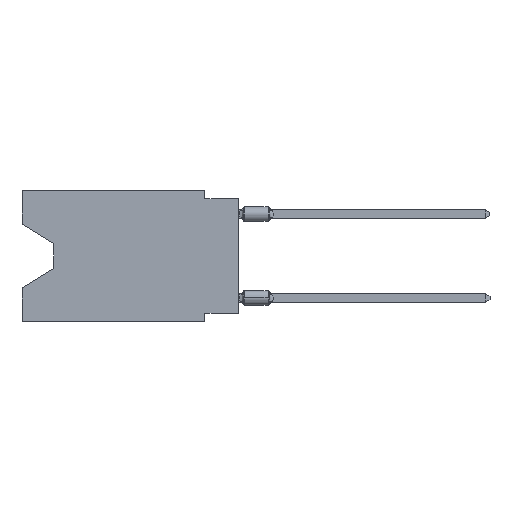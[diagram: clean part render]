
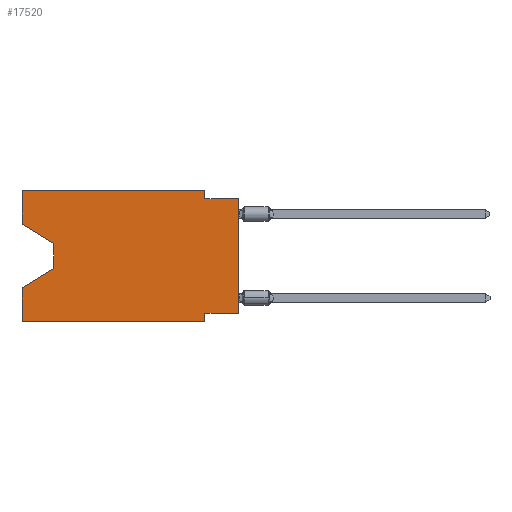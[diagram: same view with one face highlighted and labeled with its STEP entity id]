
A CAD part, left-side view. The second image highlights one B-rep face of the part: STEP entity #17520.
In plain terms, the highlighted planar face has unit normal (-1, 0, 0).
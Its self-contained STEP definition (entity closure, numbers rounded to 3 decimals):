
#635 = CARTESIAN_POINT ( 'NONE',  ( 0., 13.97, -5.893 ) ) ;
#1860 = CARTESIAN_POINT ( 'NONE',  ( 0., 0., 0. ) ) ;
#1913 = LINE ( 'NONE', #5358, #4241 ) ;
#2223 = CARTESIAN_POINT ( 'NONE',  ( 0., 16.383, -9.906 ) ) ;
#2336 = DIRECTION ( 'NONE',  ( 0., -1., 0. ) ) ;
#2505 = DIRECTION ( 'NONE',  ( 0., 0., 1. ) ) ;
#2798 = VECTOR ( 'NONE', #19032, 1000. ) ;
#3172 = ORIENTED_EDGE ( 'NONE', *, *, #19036, .T. ) ;
#3217 = EDGE_CURVE ( 'NONE', #8959, #5045, #1913, .T. ) ;
#3568 = DIRECTION ( 'NONE',  ( 0., -1., 0. ) ) ;
#4062 = DIRECTION ( 'NONE',  ( 1., 0., 0. ) ) ;
#4241 = VECTOR ( 'NONE', #5244, 1000. ) ;
#4574 = CARTESIAN_POINT ( 'NONE',  ( 0., 2.54, -9.906 ) ) ;
#4820 = CARTESIAN_POINT ( 'NONE',  ( 0., 13.97, -5.893 ) ) ;
#4947 = EDGE_CURVE ( 'NONE', #20258, #6249, #11176, .T. ) ;
#5045 = VERTEX_POINT ( 'NONE', #15097 ) ;
#5244 = DIRECTION ( 'NONE',  ( 0., 0., -1. ) ) ;
#5317 = VERTEX_POINT ( 'NONE', #7220 ) ;
#5358 = CARTESIAN_POINT ( 'NONE',  ( 0., 2.54, 0. ) ) ;
#5420 = LINE ( 'NONE', #1860, #16963 ) ;
#5758 = VECTOR ( 'NONE', #14984, 1000. ) ;
#5799 = PLANE ( 'NONE',  #7624 ) ;
#5903 = CARTESIAN_POINT ( 'NONE',  ( 0., 13.97, -4.013 ) ) ;
#6205 = VERTEX_POINT ( 'NONE', #11636 ) ;
#6249 = VERTEX_POINT ( 'NONE', #9445 ) ;
#6511 = CARTESIAN_POINT ( 'NONE',  ( 0., 16.383, -7.36 ) ) ;
#7022 = LINE ( 'NONE', #19379, #10149 ) ;
#7165 = CARTESIAN_POINT ( 'NONE',  ( 0., 0., -9.271 ) ) ;
#7220 = CARTESIAN_POINT ( 'NONE',  ( 0., 16.383, -2.546 ) ) ;
#7221 = VECTOR ( 'NONE', #15803, 1000. ) ;
#7257 = CARTESIAN_POINT ( 'NONE',  ( 0., 0., -0.635 ) ) ;
#7326 = VECTOR ( 'NONE', #2336, 1000. ) ;
#7369 = EDGE_CURVE ( 'NONE', #6205, #18120, #13183, .T. ) ;
#7464 = EDGE_CURVE ( 'NONE', #16154, #20258, #20544, .T. ) ;
#7595 = ORIENTED_EDGE ( 'NONE', *, *, #7369, .T. ) ;
#7624 = AXIS2_PLACEMENT_3D ( 'NONE', #19879, #4062, #11342 ) ;
#7678 = EDGE_CURVE ( 'NONE', #5045, #13814, #17535, .T. ) ;
#7710 = EDGE_CURVE ( 'NONE', #18779, #8959, #7022, .T. ) ;
#8102 = ORIENTED_EDGE ( 'NONE', *, *, #4947, .F. ) ;
#8224 = EDGE_CURVE ( 'NONE', #10060, #6249, #10991, .T. ) ;
#8227 = ORIENTED_EDGE ( 'NONE', *, *, #7464, .F. ) ;
#8959 = VERTEX_POINT ( 'NONE', #9063 ) ;
#9063 = CARTESIAN_POINT ( 'NONE',  ( 0., 2.54, 0. ) ) ;
#9262 = FACE_OUTER_BOUND ( 'NONE', #15163, .T. ) ;
#9445 = CARTESIAN_POINT ( 'NONE',  ( 0., 2.54, -9.906 ) ) ;
#10060 = VERTEX_POINT ( 'NONE', #19247 ) ;
#10149 = VECTOR ( 'NONE', #3568, 1000. ) ;
#10896 = VECTOR ( 'NONE', #21465, 1000. ) ;
#10991 = LINE ( 'NONE', #2223, #7326 ) ;
#11176 = LINE ( 'NONE', #4574, #5758 ) ;
#11342 = DIRECTION ( 'NONE',  ( 0., 0., -1. ) ) ;
#11347 = CARTESIAN_POINT ( 'NONE',  ( 0., 16.383, 0. ) ) ;
#11468 = LINE ( 'NONE', #635, #16422 ) ;
#11636 = CARTESIAN_POINT ( 'NONE',  ( 0., 13.97, -4.013 ) ) ;
#11999 = CARTESIAN_POINT ( 'NONE',  ( 0., 0., -9.271 ) ) ;
#12060 = ORIENTED_EDGE ( 'NONE', *, *, #7710, .F. ) ;
#12657 = CARTESIAN_POINT ( 'NONE',  ( 0., 16.383, 0. ) ) ;
#12980 = DIRECTION ( 'NONE',  ( 0., 0.855, -0.519 ) ) ;
#13183 = LINE ( 'NONE', #5903, #10896 ) ;
#13571 = EDGE_CURVE ( 'NONE', #10060, #14639, #14663, .T. ) ;
#13605 = CARTESIAN_POINT ( 'NONE',  ( 0., 2.54, -9.271 ) ) ;
#13814 = VERTEX_POINT ( 'NONE', #19246 ) ;
#14447 = ORIENTED_EDGE ( 'NONE', *, *, #3217, .F. ) ;
#14639 = VERTEX_POINT ( 'NONE', #6511 ) ;
#14663 = LINE ( 'NONE', #19295, #16041 ) ;
#14984 = DIRECTION ( 'NONE',  ( 0., 0., -1. ) ) ;
#15097 = CARTESIAN_POINT ( 'NONE',  ( 0., 2.54, -0.635 ) ) ;
#15163 = EDGE_LOOP ( 'NONE', ( #22680, #7595, #21124, #19895, #18782, #8102, #8227, #3172, #15219, #14447, #12060, #18870 ) ) ;
#15219 = ORIENTED_EDGE ( 'NONE', *, *, #7678, .F. ) ;
#15803 = DIRECTION ( 'NONE',  ( 0., -1., 0. ) ) ;
#15966 = EDGE_CURVE ( 'NONE', #18120, #14639, #11468, .T. ) ;
#16041 = VECTOR ( 'NONE', #19851, 1000. ) ;
#16154 = VERTEX_POINT ( 'NONE', #7165 ) ;
#16422 = VECTOR ( 'NONE', #12980, 1000. ) ;
#16855 = VECTOR ( 'NONE', #18506, 1000. ) ;
#16963 = VECTOR ( 'NONE', #17768, 1000. ) ;
#17520 = ADVANCED_FACE ( 'NONE', ( #9262 ), #5799, .F. ) ;
#17535 = LINE ( 'NONE', #7257, #7221 ) ;
#17768 = DIRECTION ( 'NONE',  ( 0., 0., 1. ) ) ;
#18120 = VERTEX_POINT ( 'NONE', #4820 ) ;
#18506 = DIRECTION ( 'NONE',  ( 0., -0.855, -0.519 ) ) ;
#18779 = VERTEX_POINT ( 'NONE', #11347 ) ;
#18782 = ORIENTED_EDGE ( 'NONE', *, *, #8224, .T. ) ;
#18870 = ORIENTED_EDGE ( 'NONE', *, *, #20464, .F. ) ;
#19032 = DIRECTION ( 'NONE',  ( 0., 1., 0. ) ) ;
#19036 = EDGE_CURVE ( 'NONE', #16154, #13814, #5420, .T. ) ;
#19246 = CARTESIAN_POINT ( 'NONE',  ( 0., 0., -0.635 ) ) ;
#19247 = CARTESIAN_POINT ( 'NONE',  ( 0., 16.383, -9.906 ) ) ;
#19295 = CARTESIAN_POINT ( 'NONE',  ( 0., 16.383, 0. ) ) ;
#19379 = CARTESIAN_POINT ( 'NONE',  ( 0., 16.383, 0. ) ) ;
#19815 = LINE ( 'NONE', #12657, #19956 ) ;
#19851 = DIRECTION ( 'NONE',  ( 0., 0., 1. ) ) ;
#19879 = CARTESIAN_POINT ( 'NONE',  ( 0., 16.383, 0. ) ) ;
#19895 = ORIENTED_EDGE ( 'NONE', *, *, #13571, .F. ) ;
#19956 = VECTOR ( 'NONE', #2505, 1000. ) ;
#20258 = VERTEX_POINT ( 'NONE', #13605 ) ;
#20464 = EDGE_CURVE ( 'NONE', #5317, #18779, #19815, .T. ) ;
#20544 = LINE ( 'NONE', #11999, #2798 ) ;
#20585 = LINE ( 'NONE', #22074, #16855 ) ;
#21124 = ORIENTED_EDGE ( 'NONE', *, *, #15966, .T. ) ;
#21465 = DIRECTION ( 'NONE',  ( 0., 0., -1. ) ) ;
#22074 = CARTESIAN_POINT ( 'NONE',  ( 0., 16.383, -2.546 ) ) ;
#22269 = EDGE_CURVE ( 'NONE', #5317, #6205, #20585, .T. ) ;
#22680 = ORIENTED_EDGE ( 'NONE', *, *, #22269, .T. ) ;
